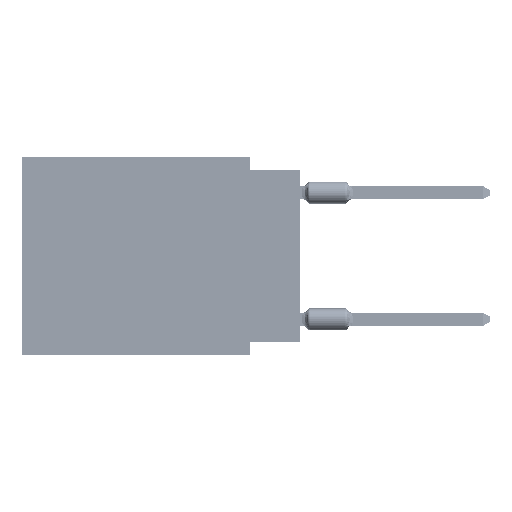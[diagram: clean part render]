
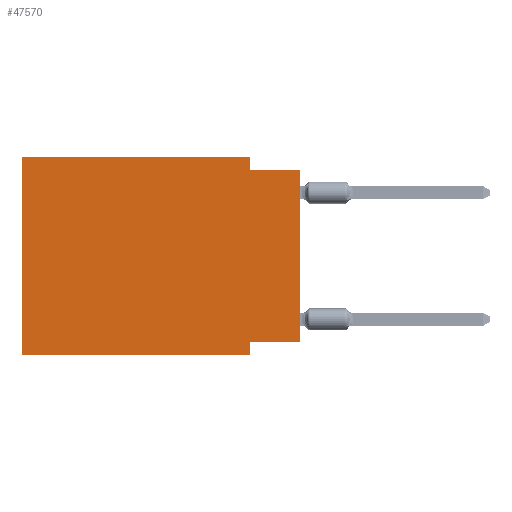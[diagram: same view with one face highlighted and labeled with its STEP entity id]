
A CAD part, left-side view. The second image highlights one B-rep face of the part: STEP entity #47570.
In plain terms, the highlighted planar face has unit normal (-1, 0, 0).
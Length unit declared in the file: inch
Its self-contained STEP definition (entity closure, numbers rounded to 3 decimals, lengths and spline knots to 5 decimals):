
#189 = DIRECTION ( 'NONE',  ( 0., 1., 0. ) ) ;
#1692 = ORIENTED_EDGE ( 'NONE', *, *, #9541, .F. ) ;
#2287 = VECTOR ( 'NONE', #31242, 39.37008 ) ;
#3199 = ORIENTED_EDGE ( 'NONE', *, *, #31977, .T. ) ;
#3597 = CARTESIAN_POINT ( 'NONE',  ( 0., 0.55, 0. ) ) ;
#3600 = EDGE_LOOP ( 'NONE', ( #29585, #1692, #47536, #50985, #45717, #3199, #45124, #50396 ) ) ;
#6251 = LINE ( 'NONE', #46209, #33832 ) ;
#8390 = LINE ( 'NONE', #9098, #2287 ) ;
#9098 = CARTESIAN_POINT ( 'NONE',  ( 0., 0.1, -0.39 ) ) ;
#9110 = DIRECTION ( 'NONE',  ( 0., 0., -1. ) ) ;
#9541 = EDGE_CURVE ( 'NONE', #70116, #12117, #6251, .T. ) ;
#12117 = VERTEX_POINT ( 'NONE', #40606 ) ;
#17539 = VERTEX_POINT ( 'NONE', #37217 ) ;
#18264 = CARTESIAN_POINT ( 'NONE',  ( 0., 0.1, 0. ) ) ;
#19227 = LINE ( 'NONE', #3597, #24692 ) ;
#20701 = LINE ( 'NONE', #31942, #63929 ) ;
#21548 = EDGE_CURVE ( 'NONE', #40138, #71080, #50345, .T. ) ;
#23230 = CARTESIAN_POINT ( 'NONE',  ( 0., 0.55, -0.39 ) ) ;
#24692 = VECTOR ( 'NONE', #47589, 39.37008 ) ;
#24704 = DIRECTION ( 'NONE',  ( 0., 0., 1. ) ) ;
#29035 = CARTESIAN_POINT ( 'NONE',  ( 0., 0.55, 0. ) ) ;
#29585 = ORIENTED_EDGE ( 'NONE', *, *, #62127, .T. ) ;
#31242 = DIRECTION ( 'NONE',  ( 0., 0., -1. ) ) ;
#31835 = VERTEX_POINT ( 'NONE', #23230 ) ;
#31942 = CARTESIAN_POINT ( 'NONE',  ( 0., 0.55, -0.39 ) ) ;
#31977 = EDGE_CURVE ( 'NONE', #31835, #17539, #20701, .T. ) ;
#32747 = EDGE_CURVE ( 'NONE', #45869, #70116, #57980, .T. ) ;
#32829 = LINE ( 'NONE', #49554, #59680 ) ;
#33832 = VECTOR ( 'NONE', #34580, 39.37008 ) ;
#34580 = DIRECTION ( 'NONE',  ( 0., -1., 0. ) ) ;
#36316 = CARTESIAN_POINT ( 'NONE',  ( 0., 0.55, 0. ) ) ;
#37217 = CARTESIAN_POINT ( 'NONE',  ( 0., 0.1, -0.39 ) ) ;
#38925 = VERTEX_POINT ( 'NONE', #29035 ) ;
#40138 = VERTEX_POINT ( 'NONE', #43465 ) ;
#40547 = DIRECTION ( 'NONE',  ( 0., 0., -1. ) ) ;
#40606 = CARTESIAN_POINT ( 'NONE',  ( 0., 0., -0.025 ) ) ;
#41442 = DIRECTION ( 'NONE',  ( 1., 0., 0. ) ) ;
#42171 = PLANE ( 'NONE',  #43868 ) ;
#42518 = EDGE_CURVE ( 'NONE', #71080, #17539, #8390, .T. ) ;
#43465 = CARTESIAN_POINT ( 'NONE',  ( 0., 0., -0.365 ) ) ;
#43868 = AXIS2_PLACEMENT_3D ( 'NONE', #57812, #41442, #9110 ) ;
#44096 = DIRECTION ( 'NONE',  ( 0., 0., 1. ) ) ;
#45124 = ORIENTED_EDGE ( 'NONE', *, *, #42518, .F. ) ;
#45717 = ORIENTED_EDGE ( 'NONE', *, *, #53705, .F. ) ;
#45869 = VERTEX_POINT ( 'NONE', #18264 ) ;
#46209 = CARTESIAN_POINT ( 'NONE',  ( 0., 0., -0.025 ) ) ;
#47536 = ORIENTED_EDGE ( 'NONE', *, *, #32747, .F. ) ;
#47570 = ADVANCED_FACE ( 'NONE', ( #52365 ), #42171, .F. ) ;
#47589 = DIRECTION ( 'NONE',  ( 0., -1., 0. ) ) ;
#47963 = VECTOR ( 'NONE', #40547, 39.37008 ) ;
#49554 = CARTESIAN_POINT ( 'NONE',  ( 0., 0., 0. ) ) ;
#50345 = LINE ( 'NONE', #62306, #59597 ) ;
#50396 = ORIENTED_EDGE ( 'NONE', *, *, #21548, .F. ) ;
#50985 = ORIENTED_EDGE ( 'NONE', *, *, #56794, .F. ) ;
#52365 = FACE_OUTER_BOUND ( 'NONE', #3600, .T. ) ;
#53705 = EDGE_CURVE ( 'NONE', #31835, #38925, #58494, .T. ) ;
#54122 = DIRECTION ( 'NONE',  ( 0., -1., 0. ) ) ;
#56794 = EDGE_CURVE ( 'NONE', #38925, #45869, #19227, .T. ) ;
#57812 = CARTESIAN_POINT ( 'NONE',  ( 0., 0.55, 0. ) ) ;
#57980 = LINE ( 'NONE', #68893, #47963 ) ;
#58494 = LINE ( 'NONE', #36316, #60520 ) ;
#59597 = VECTOR ( 'NONE', #189, 39.37008 ) ;
#59680 = VECTOR ( 'NONE', #44096, 39.37008 ) ;
#60520 = VECTOR ( 'NONE', #24704, 39.37008 ) ;
#62127 = EDGE_CURVE ( 'NONE', #40138, #12117, #32829, .T. ) ;
#62306 = CARTESIAN_POINT ( 'NONE',  ( 0., 0., -0.365 ) ) ;
#63929 = VECTOR ( 'NONE', #54122, 39.37008 ) ;
#66379 = CARTESIAN_POINT ( 'NONE',  ( 0., 0.1, -0.365 ) ) ;
#68893 = CARTESIAN_POINT ( 'NONE',  ( 0., 0.1, 0. ) ) ;
#69579 = CARTESIAN_POINT ( 'NONE',  ( 0., 0.1, -0.025 ) ) ;
#70116 = VERTEX_POINT ( 'NONE', #69579 ) ;
#71080 = VERTEX_POINT ( 'NONE', #66379 ) ;
